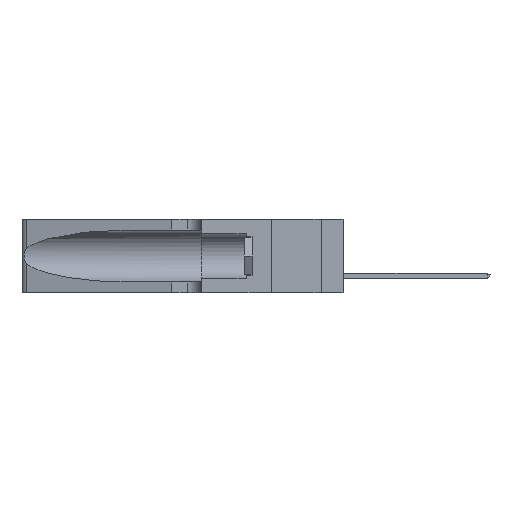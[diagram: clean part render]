
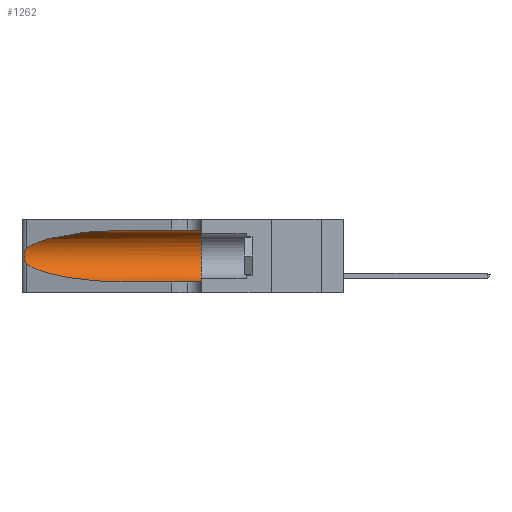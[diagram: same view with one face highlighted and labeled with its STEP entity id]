
A CAD part, left-side view. The second image highlights one B-rep face of the part: STEP entity #1262.
In plain terms, the highlighted cylindrical face has radius 3.308 mm (diameter 6.617 mm), a partial arc.
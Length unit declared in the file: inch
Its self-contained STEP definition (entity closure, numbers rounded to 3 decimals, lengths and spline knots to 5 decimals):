
#37 = VERTEX_POINT ( 'NONE', #8076 ) ;
#162 = CARTESIAN_POINT ( 'NONE',  ( 0.1305, 0.72297, 0.05475 ) ) ;
#257 = FACE_OUTER_BOUND ( 'NONE', #15080, .T. ) ;
#855 = CARTESIAN_POINT ( 'NONE',  ( 0.1305, 0.72297, 0.31525 ) ) ;
#1019 = CARTESIAN_POINT ( 'NONE',  ( 0.1305, 1.61858, 0.185 ) ) ;
#1262 = ADVANCED_FACE ( 'NONE', ( #257 ), #4609, .F. ) ;
#2031 =( BOUNDED_CURVE ( )  B_SPLINE_CURVE ( 3, ( #21503, #13515, #15536, #3637 ),
 .UNSPECIFIED., .F., .T. ) 
 B_SPLINE_CURVE_WITH_KNOTS ( ( 4, 4 ),
 ( 3.44316, 4.71239 ),
 .UNSPECIFIED. ) 
 CURVE ( )  GEOMETRIC_REPRESENTATION_ITEM ( )  RATIONAL_B_SPLINE_CURVE ( ( 1., 0.87, 0.87, 1. ) ) 
 REPRESENTATION_ITEM ( '' )  );
#2719 = CARTESIAN_POINT ( 'NONE',  ( 0.25555, 1.22994, 0.2215 ) ) ;
#2803 = CARTESIAN_POINT ( 'NONE',  ( 0.26075, 1.23896, 0.19203 ) ) ;
#2874 = CARTESIAN_POINT ( 'NONE',  ( 0.18966, 0.96281, 0.31525 ) ) ;
#3055 = CARTESIAN_POINT ( 'NONE',  ( 0.25487, 1.22718, 0.22369 ) ) ;
#3263 = VECTOR ( 'NONE', #16903, 39.37008 ) ;
#3600 = ORIENTED_EDGE ( 'NONE', *, *, #17129, .F. ) ;
#3627 = CARTESIAN_POINT ( 'NONE',  ( 0.1305, 0.35, 0.185 ) ) ;
#3637 = CARTESIAN_POINT ( 'NONE',  ( 0.1305, 0.72297, 0.05475 ) ) ;
#3787 = VERTEX_POINT ( 'NONE', #7913 ) ;
#3920 = LINE ( 'NONE', #10382, #24413 ) ;
#4210 = DIRECTION ( 'NONE',  ( 0., -1., 0. ) ) ;
#4499 = VERTEX_POINT ( 'NONE', #24235 ) ;
#4609 = CYLINDRICAL_SURFACE ( 'NONE', #16826, 0.13025 ) ;
#4887 = CARTESIAN_POINT ( 'NONE',  ( 0.25854, 1.2359, 0.20912 ) ) ;
#6640 =( BOUNDED_CURVE ( )  B_SPLINE_CURVE ( 3, ( #24659, #2874, #8874, #3055 ),
 .UNSPECIFIED., .F., .T. ) 
 B_SPLINE_CURVE_WITH_KNOTS ( ( 4, 4 ),
 ( 1.5708, 2.84003 ),
 .UNSPECIFIED. ) 
 CURVE ( )  GEOMETRIC_REPRESENTATION_ITEM ( )  RATIONAL_B_SPLINE_CURVE ( ( 1., 0.87, 0.87, 1. ) ) 
 REPRESENTATION_ITEM ( '' )  );
#7356 = ORIENTED_EDGE ( 'NONE', *, *, #23762, .T. ) ;
#7649 = ORIENTED_EDGE ( 'NONE', *, *, #14263, .T. ) ;
#7913 = CARTESIAN_POINT ( 'NONE',  ( 0.1305, 0.35, 0.31525 ) ) ;
#8076 = CARTESIAN_POINT ( 'NONE',  ( 0.25487, 1.22718, 0.22369 ) ) ;
#8264 = DIRECTION ( 'NONE',  ( 0., 0., 1. ) ) ;
#8501 = ORIENTED_EDGE ( 'NONE', *, *, #11605, .F. ) ;
#8698 = CARTESIAN_POINT ( 'NONE',  ( 0.25639, 1.23184, 0.21858 ) ) ;
#8781 = CARTESIAN_POINT ( 'NONE',  ( 0.26075, 1.23896, 0.178 ) ) ;
#8874 = CARTESIAN_POINT ( 'NONE',  ( 0.2373, 1.15595, 0.28018 ) ) ;
#10281 = CARTESIAN_POINT ( 'NONE',  ( 0.25639, 1.23186, 0.15144 ) ) ;
#10290 = DIRECTION ( 'NONE',  ( 0., 1., 0. ) ) ;
#10382 = CARTESIAN_POINT ( 'NONE',  ( 0.1305, 1.61858, 0.05475 ) ) ;
#11605 = EDGE_CURVE ( 'NONE', #3787, #4499, #24882, .T. ) ;
#12090 = VERTEX_POINT ( 'NONE', #21230 ) ;
#12131 = ORIENTED_EDGE ( 'NONE', *, *, #16694, .T. ) ;
#12674 = CARTESIAN_POINT ( 'NONE',  ( 0.26018, 1.23835, 0.19895 ) ) ;
#12725 = VERTEX_POINT ( 'NONE', #855 ) ;
#12953 = CARTESIAN_POINT ( 'NONE',  ( 0.1305, 1.61858, 0.31525 ) ) ;
#13292 = EDGE_CURVE ( 'NONE', #37, #12090, #15072, .T. ) ;
#13515 = CARTESIAN_POINT ( 'NONE',  ( 0.2373, 1.15595, 0.08982 ) ) ;
#14263 = EDGE_CURVE ( 'NONE', #16524, #4499, #3920, .T. ) ;
#14780 = CARTESIAN_POINT ( 'NONE',  ( 0.25487, 1.22718, 0.22369 ) ) ;
#15072 = B_SPLINE_CURVE_WITH_KNOTS ( 'NONE', 3,
 ( #14780, #2719, #8698, #22624, #4887, #12674, #2803, #8781, #22701, #21455, #16944, #10281, #22820, #20239 ),
 .UNSPECIFIED., .F., .F.,
 ( 4, 2, 2, 2, 2, 2, 4 ),
 ( 0., 0.00027, 0.00053, 0.00107, 0.0016, 0.00187, 0.00214 ),
 .UNSPECIFIED. ) ;
#15080 = EDGE_LOOP ( 'NONE', ( #7356, #22024, #12131, #7649, #8501, #3600 ) ) ;
#15536 = CARTESIAN_POINT ( 'NONE',  ( 0.18966, 0.96281, 0.05475 ) ) ;
#16524 = VERTEX_POINT ( 'NONE', #162 ) ;
#16694 = EDGE_CURVE ( 'NONE', #12090, #16524, #2031, .T. ) ;
#16826 = AXIS2_PLACEMENT_3D ( 'NONE', #1019, #24332, #19349 ) ;
#16903 = DIRECTION ( 'NONE',  ( 0., -1., 0. ) ) ;
#16944 = CARTESIAN_POINT ( 'NONE',  ( 0.25789, 1.23486, 0.15765 ) ) ;
#17129 = EDGE_CURVE ( 'NONE', #12725, #3787, #17589, .T. ) ;
#17589 = LINE ( 'NONE', #12953, #3263 ) ;
#19349 = DIRECTION ( 'NONE',  ( 0., 0., -1. ) ) ;
#19620 = AXIS2_PLACEMENT_3D ( 'NONE', #3627, #10290, #8264 ) ;
#20239 = CARTESIAN_POINT ( 'NONE',  ( 0.25487, 1.22718, 0.14631 ) ) ;
#21230 = CARTESIAN_POINT ( 'NONE',  ( 0.25487, 1.22718, 0.14631 ) ) ;
#21455 = CARTESIAN_POINT ( 'NONE',  ( 0.25856, 1.23593, 0.16098 ) ) ;
#21503 = CARTESIAN_POINT ( 'NONE',  ( 0.25487, 1.22718, 0.14631 ) ) ;
#22024 = ORIENTED_EDGE ( 'NONE', *, *, #13292, .T. ) ;
#22624 = CARTESIAN_POINT ( 'NONE',  ( 0.25787, 1.23484, 0.2124 ) ) ;
#22701 = CARTESIAN_POINT ( 'NONE',  ( 0.26017, 1.23833, 0.17102 ) ) ;
#22820 = CARTESIAN_POINT ( 'NONE',  ( 0.25555, 1.22993, 0.14849 ) ) ;
#23762 = EDGE_CURVE ( 'NONE', #12725, #37, #6640, .T. ) ;
#24235 = CARTESIAN_POINT ( 'NONE',  ( 0.1305, 0.35, 0.05475 ) ) ;
#24332 = DIRECTION ( 'NONE',  ( 0., -1., 0. ) ) ;
#24413 = VECTOR ( 'NONE', #4210, 39.37008 ) ;
#24659 = CARTESIAN_POINT ( 'NONE',  ( 0.1305, 0.72297, 0.31525 ) ) ;
#24882 = CIRCLE ( 'NONE', #19620, 0.13025 ) ;
